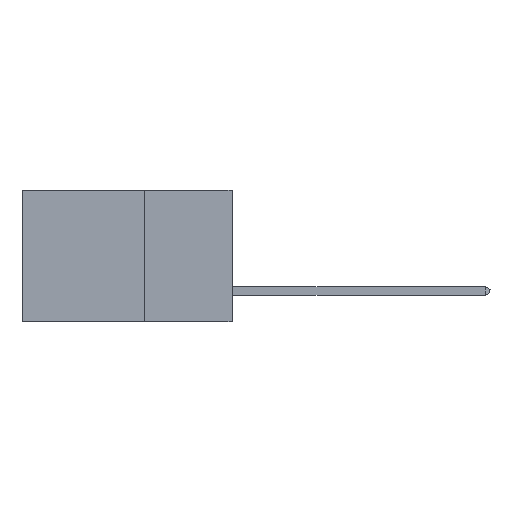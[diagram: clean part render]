
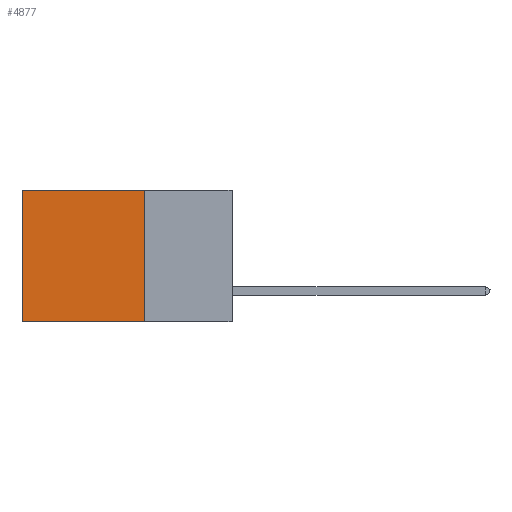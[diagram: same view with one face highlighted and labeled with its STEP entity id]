
A CAD part, left-side view. The second image highlights one B-rep face of the part: STEP entity #4877.
In plain terms, the highlighted planar face has unit normal (-1, 0, 0).
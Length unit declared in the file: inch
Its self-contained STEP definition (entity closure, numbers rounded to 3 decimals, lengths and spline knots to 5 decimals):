
#667 = DIRECTION ( 'NONE',  ( 0., 0., -1. ) ) ;
#1579 = DIRECTION ( 'NONE',  ( 0., 1., 0. ) ) ;
#2201 = CARTESIAN_POINT ( 'NONE',  ( 0.2875, 0.25, -0.375 ) ) ;
#2748 = ORIENTED_EDGE ( 'NONE', *, *, #13800, .F. ) ;
#3741 = CARTESIAN_POINT ( 'NONE',  ( 0.2875, 0.25, -0.375 ) ) ;
#4877 = ADVANCED_FACE ( 'NONE', ( #14169 ), #5128, .F. ) ;
#4954 = ORIENTED_EDGE ( 'NONE', *, *, #16151, .F. ) ;
#5128 = PLANE ( 'NONE',  #13022 ) ;
#5889 = EDGE_CURVE ( 'NONE', #7970, #10900, #15231, .T. ) ;
#6922 = ORIENTED_EDGE ( 'NONE', *, *, #11198, .T. ) ;
#7373 = CARTESIAN_POINT ( 'NONE',  ( 0.2875, 0.25, -0.375 ) ) ;
#7723 = CARTESIAN_POINT ( 'NONE',  ( 0.2875, 0.6, -0.375 ) ) ;
#7970 = VERTEX_POINT ( 'NONE', #9819 ) ;
#8233 = CARTESIAN_POINT ( 'NONE',  ( 0.2875, 0.25, -0.375 ) ) ;
#8295 = VECTOR ( 'NONE', #17146, 39.37008 ) ;
#8952 = LINE ( 'NONE', #2201, #14364 ) ;
#9819 = CARTESIAN_POINT ( 'NONE',  ( 0.2875, 0.6, 0. ) ) ;
#10019 = CARTESIAN_POINT ( 'NONE',  ( 0.2875, 0.6, -0.375 ) ) ;
#10900 = VERTEX_POINT ( 'NONE', #7723 ) ;
#11198 = EDGE_CURVE ( 'NONE', #15569, #7970, #11199, .T. ) ;
#11199 = LINE ( 'NONE', #14022, #12948 ) ;
#11513 = VECTOR ( 'NONE', #667, 39.37008 ) ;
#11918 = DIRECTION ( 'NONE',  ( 0., 1., 0. ) ) ;
#12030 = DIRECTION ( 'NONE',  ( 1., 0., 0. ) ) ;
#12491 = EDGE_LOOP ( 'NONE', ( #13082, #4954, #2748, #6922 ) ) ;
#12948 = VECTOR ( 'NONE', #1579, 39.37008 ) ;
#13022 = AXIS2_PLACEMENT_3D ( 'NONE', #3741, #12030, #14815 ) ;
#13082 = ORIENTED_EDGE ( 'NONE', *, *, #5889, .T. ) ;
#13800 = EDGE_CURVE ( 'NONE', #15569, #15761, #15678, .T. ) ;
#14022 = CARTESIAN_POINT ( 'NONE',  ( 0.2875, 0.25, 0. ) ) ;
#14169 = FACE_OUTER_BOUND ( 'NONE', #12491, .T. ) ;
#14364 = VECTOR ( 'NONE', #11918, 39.37008 ) ;
#14815 = DIRECTION ( 'NONE',  ( 0., 0., -1. ) ) ;
#14973 = CARTESIAN_POINT ( 'NONE',  ( 0.2875, 0.25, 0. ) ) ;
#15231 = LINE ( 'NONE', #10019, #11513 ) ;
#15569 = VERTEX_POINT ( 'NONE', #14973 ) ;
#15678 = LINE ( 'NONE', #7373, #8295 ) ;
#15761 = VERTEX_POINT ( 'NONE', #8233 ) ;
#16151 = EDGE_CURVE ( 'NONE', #15761, #10900, #8952, .T. ) ;
#17146 = DIRECTION ( 'NONE',  ( 0., 0., -1. ) ) ;
